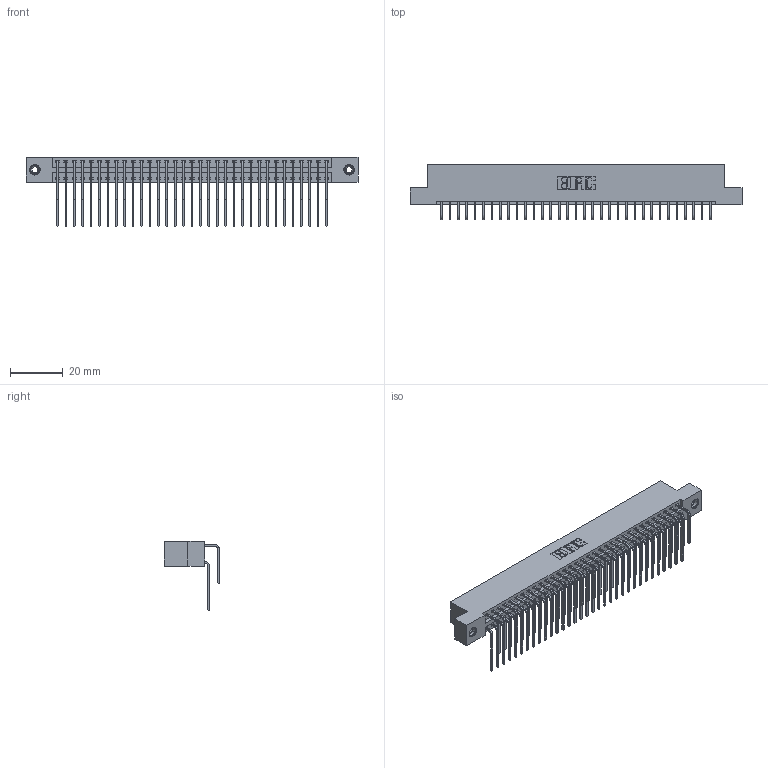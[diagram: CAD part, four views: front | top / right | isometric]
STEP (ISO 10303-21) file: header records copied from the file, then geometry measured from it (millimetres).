
FILE_DESCRIPTION (( 'STEP AP203' ), '1' );
FILE_NAME ('346-066-559-208.STEP', '2022-05-24T18:06:27', ( '' ), ( '' ), 'SwSTEP 2.0', 'SolidWorks 2020', '' );
FILE_SCHEMA (( 'CONFIG_CONTROL_DESIGN' ));
Length unit declared in the file: inch
Products named in the file (5): 346-066-559-208; 346 Part_Flush Mounting Lugs - 0.156 Dia-TI; 345-292-001_558 559 Tail - 1; 345-250-001_345-250-003-102; 345-292-001_559 Tail - 2
Assembly tree (69 placements, depth 2):
  346-066-559-208
    346 Part_Flush Mounting Lugs - 0.156 Dia-TI
    345-292-001_558 559 Tail - 1  x33
    345-292-001_559 Tail - 2  x33
    345-250-001_345-250-003-102  x2
Bounding box: 125.35 x 20.89 x 26.16 mm (x, y, z)
Volume: 12527.4 mm3; surface area: 18924.9 mm2
Topology: 69 solids, 69 shells, 3746 faces, 11091 edges, 7298 vertices
Faces by surface type: plane 2550, cylinder 1180, cone 12, torus 4
Entity records: 25718 total; most frequent: CARTESIAN_POINT 4286, ORIENTED_EDGE 4162, DIRECTION 3827, EDGE_CURVE 2081, VECTOR 1757, LINE 1757, VERTEX_POINT 1380, AXIS2_PLACEMENT_3D 1035
